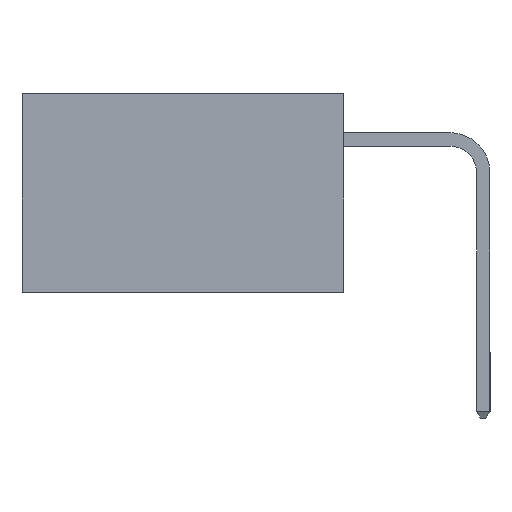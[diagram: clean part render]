
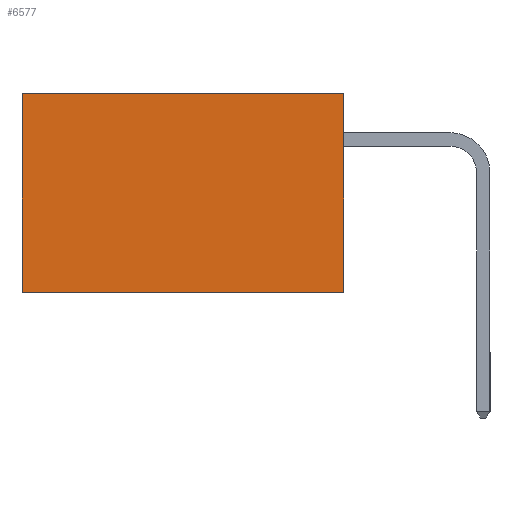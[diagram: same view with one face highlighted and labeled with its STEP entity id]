
A CAD part, left-side view. The second image highlights one B-rep face of the part: STEP entity #6577.
In plain terms, the highlighted planar face has unit normal (-1, 0, 0).
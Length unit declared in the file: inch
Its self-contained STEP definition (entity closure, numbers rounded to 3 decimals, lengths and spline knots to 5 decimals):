
#36 = DIRECTION ( 'NONE',  ( 1., 0., 0. ) ) ;
#495 = LINE ( 'NONE', #4353, #3559 ) ;
#1343 = ORIENTED_EDGE ( 'NONE', *, *, #7836, .T. ) ;
#1424 = CARTESIAN_POINT ( 'NONE',  ( 0.298, 0., -0.37 ) ) ;
#1524 = CARTESIAN_POINT ( 'NONE',  ( 0.298, 0., 0. ) ) ;
#1583 = DIRECTION ( 'NONE',  ( 0., 1., 0. ) ) ;
#1803 = PLANE ( 'NONE',  #11566 ) ;
#2747 = VERTEX_POINT ( 'NONE', #10299 ) ;
#2900 = LINE ( 'NONE', #1424, #6619 ) ;
#3454 = DIRECTION ( 'NONE',  ( 0., 0., -1. ) ) ;
#3496 = VECTOR ( 'NONE', #4960, 39.37008 ) ;
#3556 = VERTEX_POINT ( 'NONE', #3820 ) ;
#3559 = VECTOR ( 'NONE', #1583, 39.37008 ) ;
#3820 = CARTESIAN_POINT ( 'NONE',  ( 0.298, 0., -0.37 ) ) ;
#3849 = CARTESIAN_POINT ( 'NONE',  ( 0.298, 0.6, 0. ) ) ;
#4076 = ORIENTED_EDGE ( 'NONE', *, *, #7041, .F. ) ;
#4353 = CARTESIAN_POINT ( 'NONE',  ( 0.298, 0., 0. ) ) ;
#4633 = ORIENTED_EDGE ( 'NONE', *, *, #4819, .T. ) ;
#4798 = CARTESIAN_POINT ( 'NONE',  ( 0.298, 0.6, 0. ) ) ;
#4819 = EDGE_CURVE ( 'NONE', #8416, #2747, #11462, .T. ) ;
#4960 = DIRECTION ( 'NONE',  ( 0., 0., -1. ) ) ;
#5393 = DIRECTION ( 'NONE',  ( 0., 1., 0. ) ) ;
#6577 = ADVANCED_FACE ( 'NONE', ( #10836 ), #1803, .F. ) ;
#6619 = VECTOR ( 'NONE', #5393, 39.37008 ) ;
#6717 = EDGE_CURVE ( 'NONE', #3556, #2747, #2900, .T. ) ;
#7041 = EDGE_CURVE ( 'NONE', #10196, #3556, #11822, .T. ) ;
#7836 = EDGE_CURVE ( 'NONE', #10196, #8416, #495, .T. ) ;
#8056 = VECTOR ( 'NONE', #3454, 39.37008 ) ;
#8416 = VERTEX_POINT ( 'NONE', #3849 ) ;
#8426 = DIRECTION ( 'NONE',  ( 0., 0., -1. ) ) ;
#8528 = ORIENTED_EDGE ( 'NONE', *, *, #6717, .F. ) ;
#10183 = CARTESIAN_POINT ( 'NONE',  ( 0.298, 0., 0. ) ) ;
#10196 = VERTEX_POINT ( 'NONE', #11698 ) ;
#10299 = CARTESIAN_POINT ( 'NONE',  ( 0.298, 0.6, -0.37 ) ) ;
#10302 = EDGE_LOOP ( 'NONE', ( #4633, #8528, #4076, #1343 ) ) ;
#10836 = FACE_OUTER_BOUND ( 'NONE', #10302, .T. ) ;
#11462 = LINE ( 'NONE', #4798, #3496 ) ;
#11566 = AXIS2_PLACEMENT_3D ( 'NONE', #10183, #36, #8426 ) ;
#11698 = CARTESIAN_POINT ( 'NONE',  ( 0.298, 0., 0. ) ) ;
#11822 = LINE ( 'NONE', #1524, #8056 ) ;
